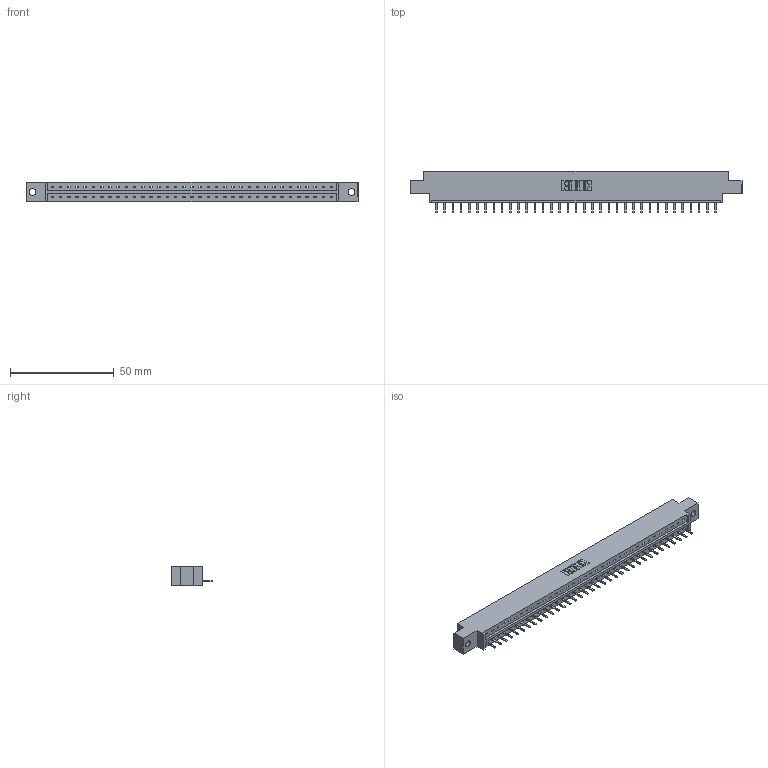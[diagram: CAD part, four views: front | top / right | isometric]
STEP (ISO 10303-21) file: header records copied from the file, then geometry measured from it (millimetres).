
FILE_DESCRIPTION (( 'STEP AP203' ), '1' );
FILE_NAME ('833-035-520-602.STEP', '2020-06-03T00:07:25', ( '' ), ( '' ), 'SwSTEP 2.0', 'SolidWorks 2020', '' );
FILE_SCHEMA (( 'CONFIG_CONTROL_DESIGN' ));
Length unit declared in the file: inch
Products named in the file (3): 833-035-520-602; 345-292-001_345-293-120; 833 Part_Offset - .128 Dia
Assembly tree (36 placements, depth 2):
  833-035-520-602
    833 Part_Offset - .128 Dia
    345-292-001_345-293-120  x35
Bounding box: 160.22 x 20.02 x 9.4 mm (x, y, z)
Volume: 15697.6 mm3; surface area: 16511.3 mm2
Topology: 36 solids, 36 shells, 2288 faces, 6763 edges, 4414 vertices
Faces by surface type: plane 1614, cylinder 674
Entity records: 22551 total; most frequent: CARTESIAN_POINT 3911, ORIENTED_EDGE 3870, DIRECTION 3301, EDGE_CURVE 1935, VECTOR 1803, LINE 1803, VERTEX_POINT 1286, AXIS2_PLACEMENT_3D 749
